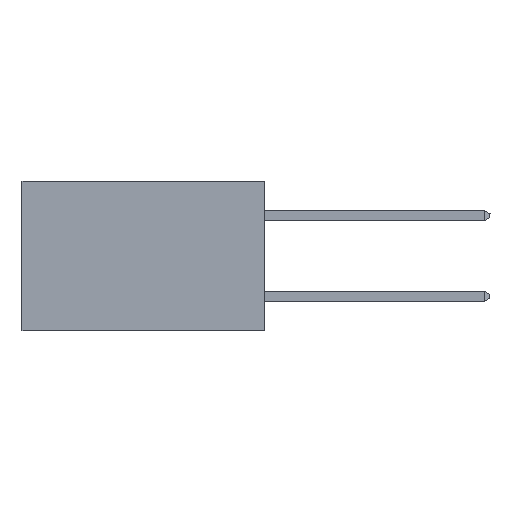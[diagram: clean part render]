
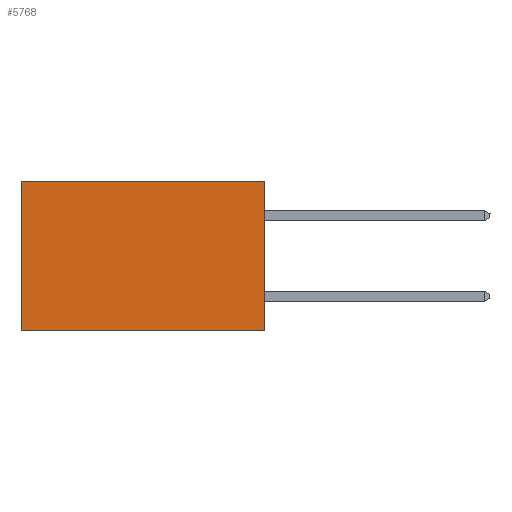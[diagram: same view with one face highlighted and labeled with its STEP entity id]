
A CAD part, left-side view. The second image highlights one B-rep face of the part: STEP entity #5768.
In plain terms, the highlighted planar face has unit normal (-1, 0, 0).
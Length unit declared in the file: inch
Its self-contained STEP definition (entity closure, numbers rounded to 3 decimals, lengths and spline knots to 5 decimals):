
#57 = ORIENTED_EDGE ( 'NONE', *, *, #9977, .F. ) ;
#1217 = DIRECTION ( 'NONE',  ( 0., 0., -1. ) ) ;
#1387 = CARTESIAN_POINT ( 'NONE',  ( 0.298, 0., 0. ) ) ;
#1776 = LINE ( 'NONE', #14625, #2457 ) ;
#1904 = LINE ( 'NONE', #24531, #14050 ) ;
#2457 = VECTOR ( 'NONE', #5911, 39.37008 ) ;
#2972 = ORIENTED_EDGE ( 'NONE', *, *, #9045, .T. ) ;
#5768 = ADVANCED_FACE ( 'NONE', ( #15458 ), #27130, .F. ) ;
#5911 = DIRECTION ( 'NONE',  ( 0., 1., 0. ) ) ;
#7556 = LINE ( 'NONE', #1387, #8551 ) ;
#7760 = CARTESIAN_POINT ( 'NONE',  ( 0.298, 0.6, 0. ) ) ;
#8551 = VECTOR ( 'NONE', #16465, 39.37008 ) ;
#9045 = EDGE_CURVE ( 'NONE', #9724, #16260, #1904, .T. ) ;
#9724 = VERTEX_POINT ( 'NONE', #7760 ) ;
#9806 = DIRECTION ( 'NONE',  ( 1., 0., 0. ) ) ;
#9977 = EDGE_CURVE ( 'NONE', #16761, #14555, #7556, .T. ) ;
#11834 = DIRECTION ( 'NONE',  ( 0., 1., 0. ) ) ;
#12243 = LINE ( 'NONE', #22859, #14973 ) ;
#12701 = CARTESIAN_POINT ( 'NONE',  ( 0.298, 0., 0. ) ) ;
#14050 = VECTOR ( 'NONE', #26792, 39.37008 ) ;
#14555 = VERTEX_POINT ( 'NONE', #14819 ) ;
#14625 = CARTESIAN_POINT ( 'NONE',  ( 0.298, 0., 0. ) ) ;
#14819 = CARTESIAN_POINT ( 'NONE',  ( 0.298, 0., -0.37 ) ) ;
#14973 = VECTOR ( 'NONE', #11834, 39.37008 ) ;
#15256 = CARTESIAN_POINT ( 'NONE',  ( 0.298, 0.6, -0.37 ) ) ;
#15458 = FACE_OUTER_BOUND ( 'NONE', #15474, .T. ) ;
#15474 = EDGE_LOOP ( 'NONE', ( #2972, #23492, #57, #17959 ) ) ;
#16260 = VERTEX_POINT ( 'NONE', #15256 ) ;
#16465 = DIRECTION ( 'NONE',  ( 0., 0., -1. ) ) ;
#16761 = VERTEX_POINT ( 'NONE', #12701 ) ;
#17959 = ORIENTED_EDGE ( 'NONE', *, *, #18017, .T. ) ;
#18017 = EDGE_CURVE ( 'NONE', #16761, #9724, #1776, .T. ) ;
#18608 = CARTESIAN_POINT ( 'NONE',  ( 0.298, 0., 0. ) ) ;
#22859 = CARTESIAN_POINT ( 'NONE',  ( 0.298, 0., -0.37 ) ) ;
#22918 = AXIS2_PLACEMENT_3D ( 'NONE', #18608, #9806, #1217 ) ;
#23492 = ORIENTED_EDGE ( 'NONE', *, *, #27514, .F. ) ;
#24531 = CARTESIAN_POINT ( 'NONE',  ( 0.298, 0.6, 0. ) ) ;
#26792 = DIRECTION ( 'NONE',  ( 0., 0., -1. ) ) ;
#27130 = PLANE ( 'NONE',  #22918 ) ;
#27514 = EDGE_CURVE ( 'NONE', #14555, #16260, #12243, .T. ) ;
